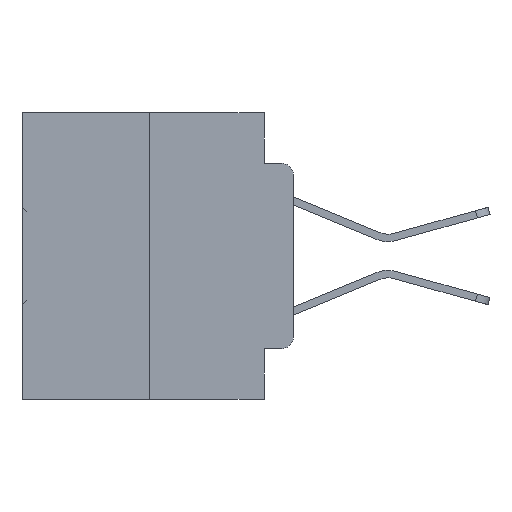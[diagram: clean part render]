
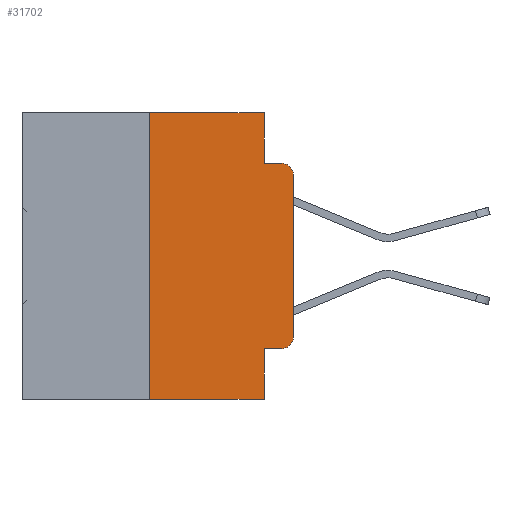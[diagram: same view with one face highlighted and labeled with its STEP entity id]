
A CAD part, left-side view. The second image highlights one B-rep face of the part: STEP entity #31702.
In plain terms, the highlighted planar face has unit normal (-1, 0, 0).
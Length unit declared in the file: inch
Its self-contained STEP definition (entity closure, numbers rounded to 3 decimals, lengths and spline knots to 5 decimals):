
#156 = AXIS2_PLACEMENT_3D ( 'NONE', #16833, #23055, #33935 ) ;
#206 = ORIENTED_EDGE ( 'NONE', *, *, #17068, .F. ) ;
#621 = LINE ( 'NONE', #27653, #10910 ) ;
#737 = DIRECTION ( 'NONE',  ( -1., 0., 0. ) ) ;
#935 = EDGE_CURVE ( 'NONE', #30131, #35096, #19298, .T. ) ;
#966 = CARTESIAN_POINT ( 'NONE',  ( 0., 0.25, 0. ) ) ;
#1275 = DIRECTION ( 'NONE',  ( 0., 0., -1. ) ) ;
#1541 = LINE ( 'NONE', #9377, #18695 ) ;
#1969 = EDGE_CURVE ( 'NONE', #28057, #4716, #1541, .T. ) ;
#1998 = LINE ( 'NONE', #12835, #2633 ) ;
#2633 = VECTOR ( 'NONE', #10178, 39.37008 ) ;
#3322 = DIRECTION ( 'NONE',  ( 0., 0., -1. ) ) ;
#3982 = AXIS2_PLACEMENT_3D ( 'NONE', #24929, #737, #1275 ) ;
#4016 = DIRECTION ( 'NONE',  ( 1., 0., 0. ) ) ;
#4716 = VERTEX_POINT ( 'NONE', #25675 ) ;
#5293 = CARTESIAN_POINT ( 'NONE',  ( 0., 0.02, -0.0885 ) ) ;
#5847 = CARTESIAN_POINT ( 'NONE',  ( 0., 0.473, 0. ) ) ;
#5877 = ORIENTED_EDGE ( 'NONE', *, *, #35123, .T. ) ;
#6029 = EDGE_CURVE ( 'NONE', #28057, #6264, #31565, .T. ) ;
#6264 = VERTEX_POINT ( 'NONE', #26720 ) ;
#7098 = DIRECTION ( 'NONE',  ( 0., 0., 1. ) ) ;
#7550 = CIRCLE ( 'NONE', #156, 0.02 ) ;
#7627 = EDGE_LOOP ( 'NONE', ( #11250, #7808, #27911, #206, #25444, #28589, #17451, #29687, #16159, #5877 ) ) ;
#7808 = ORIENTED_EDGE ( 'NONE', *, *, #935, .T. ) ;
#8125 = VECTOR ( 'NONE', #9683, 39.37008 ) ;
#8478 = VERTEX_POINT ( 'NONE', #29548 ) ;
#9377 = CARTESIAN_POINT ( 'NONE',  ( 0., 0.473, -0.5 ) ) ;
#9683 = DIRECTION ( 'NONE',  ( 0., 0., 1. ) ) ;
#9851 = DIRECTION ( 'NONE',  ( 0., 0., -1. ) ) ;
#10178 = DIRECTION ( 'NONE',  ( 0., -1., 0. ) ) ;
#10910 = VECTOR ( 'NONE', #30520, 39.37008 ) ;
#10919 = EDGE_CURVE ( 'NONE', #13749, #16878, #1998, .T. ) ;
#11250 = ORIENTED_EDGE ( 'NONE', *, *, #28331, .T. ) ;
#12171 = CARTESIAN_POINT ( 'NONE',  ( 0., 0.051, -0.0885 ) ) ;
#12511 = LINE ( 'NONE', #34245, #20146 ) ;
#12835 = CARTESIAN_POINT ( 'NONE',  ( 0., 0.051, -0.4115 ) ) ;
#13749 = VERTEX_POINT ( 'NONE', #26112 ) ;
#14487 = CARTESIAN_POINT ( 'NONE',  ( 0., 0.02, -0.4115 ) ) ;
#15128 = VERTEX_POINT ( 'NONE', #27519 ) ;
#15668 = EDGE_CURVE ( 'NONE', #18213, #35096, #621, .T. ) ;
#16159 = ORIENTED_EDGE ( 'NONE', *, *, #10919, .T. ) ;
#16833 = CARTESIAN_POINT ( 'NONE',  ( 0., 0.02, -0.3915 ) ) ;
#16878 = VERTEX_POINT ( 'NONE', #14487 ) ;
#17068 = EDGE_CURVE ( 'NONE', #15128, #18213, #12511, .T. ) ;
#17100 = VECTOR ( 'NONE', #25408, 39.37008 ) ;
#17451 = ORIENTED_EDGE ( 'NONE', *, *, #1969, .T. ) ;
#17873 = PLANE ( 'NONE',  #33588 ) ;
#18213 = VERTEX_POINT ( 'NONE', #12171 ) ;
#18695 = VECTOR ( 'NONE', #23059, 39.37008 ) ;
#19298 = CIRCLE ( 'NONE', #3982, 0.02 ) ;
#20146 = VECTOR ( 'NONE', #9851, 39.37008 ) ;
#20923 = CARTESIAN_POINT ( 'NONE',  ( 0., 0., -0.1085 ) ) ;
#23055 = DIRECTION ( 'NONE',  ( -1., 0., 0. ) ) ;
#23059 = DIRECTION ( 'NONE',  ( 0., -1., 0. ) ) ;
#24929 = CARTESIAN_POINT ( 'NONE',  ( 0., 0.02, -0.1085 ) ) ;
#25408 = DIRECTION ( 'NONE',  ( 0., -1., 0. ) ) ;
#25444 = ORIENTED_EDGE ( 'NONE', *, *, #26822, .F. ) ;
#25675 = CARTESIAN_POINT ( 'NONE',  ( 0., 0.051, -0.5 ) ) ;
#26112 = CARTESIAN_POINT ( 'NONE',  ( 0., 0.051, -0.4115 ) ) ;
#26720 = CARTESIAN_POINT ( 'NONE',  ( 0., 0.25, 0. ) ) ;
#26822 = EDGE_CURVE ( 'NONE', #6264, #15128, #27543, .T. ) ;
#27025 = CARTESIAN_POINT ( 'NONE',  ( 0., 0.25, -0.5 ) ) ;
#27519 = CARTESIAN_POINT ( 'NONE',  ( 0., 0.051, 0. ) ) ;
#27543 = LINE ( 'NONE', #5847, #17100 ) ;
#27653 = CARTESIAN_POINT ( 'NONE',  ( 0., 0.051, -0.0885 ) ) ;
#27689 = CARTESIAN_POINT ( 'NONE',  ( 0., 0.051, 0. ) ) ;
#27911 = ORIENTED_EDGE ( 'NONE', *, *, #15668, .F. ) ;
#28057 = VERTEX_POINT ( 'NONE', #27025 ) ;
#28287 = VECTOR ( 'NONE', #7098, 39.37008 ) ;
#28331 = EDGE_CURVE ( 'NONE', #8478, #30131, #31825, .T. ) ;
#28589 = ORIENTED_EDGE ( 'NONE', *, *, #6029, .F. ) ;
#28665 = EDGE_CURVE ( 'NONE', #13749, #4716, #30905, .T. ) ;
#29548 = CARTESIAN_POINT ( 'NONE',  ( 0., 0., -0.3915 ) ) ;
#29687 = ORIENTED_EDGE ( 'NONE', *, *, #28665, .F. ) ;
#30131 = VERTEX_POINT ( 'NONE', #20923 ) ;
#30520 = DIRECTION ( 'NONE',  ( 0., -1., 0. ) ) ;
#30905 = LINE ( 'NONE', #27689, #35127 ) ;
#31234 = FACE_OUTER_BOUND ( 'NONE', #7627, .T. ) ;
#31412 = DIRECTION ( 'NONE',  ( 0., 0., -1. ) ) ;
#31477 = CARTESIAN_POINT ( 'NONE',  ( 0., 0., 0. ) ) ;
#31565 = LINE ( 'NONE', #966, #8125 ) ;
#31702 = ADVANCED_FACE ( 'NONE', ( #31234 ), #17873, .F. ) ;
#31825 = LINE ( 'NONE', #31477, #28287 ) ;
#33588 = AXIS2_PLACEMENT_3D ( 'NONE', #33737, #4016, #31412 ) ;
#33737 = CARTESIAN_POINT ( 'NONE',  ( 0., 0.473, 0. ) ) ;
#33935 = DIRECTION ( 'NONE',  ( 0., 0., -1. ) ) ;
#34245 = CARTESIAN_POINT ( 'NONE',  ( 0., 0.051, 0. ) ) ;
#35096 = VERTEX_POINT ( 'NONE', #5293 ) ;
#35123 = EDGE_CURVE ( 'NONE', #16878, #8478, #7550, .T. ) ;
#35127 = VECTOR ( 'NONE', #3322, 39.37008 ) ;
